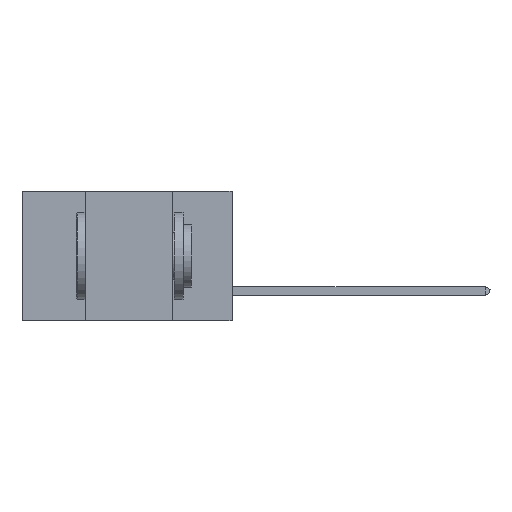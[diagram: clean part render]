
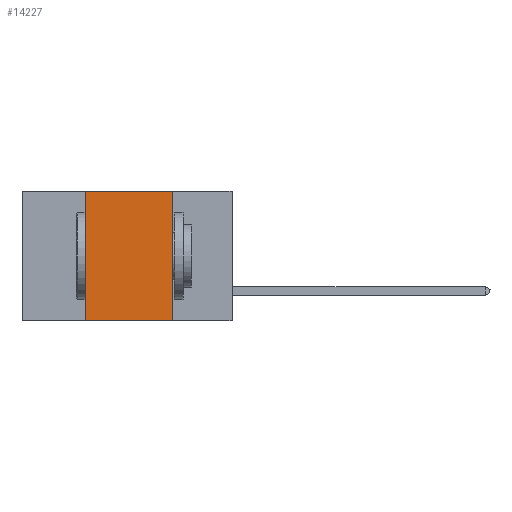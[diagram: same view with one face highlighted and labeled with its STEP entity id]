
A CAD part, left-side view. The second image highlights one B-rep face of the part: STEP entity #14227.
In plain terms, the highlighted planar face has unit normal (-1, 0, 0).
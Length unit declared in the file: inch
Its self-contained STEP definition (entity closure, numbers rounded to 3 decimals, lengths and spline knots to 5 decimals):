
#2459 = EDGE_CURVE ( 'NONE', #25816, #4849, #21942, .T. ) ;
#2851 = FACE_OUTER_BOUND ( 'NONE', #14474, .T. ) ;
#3013 = DIRECTION ( 'NONE',  ( 1., 0., 0. ) ) ;
#3848 = CARTESIAN_POINT ( 'NONE',  ( 0., 0.42, 0. ) ) ;
#4849 = VERTEX_POINT ( 'NONE', #29772 ) ;
#5055 = ORIENTED_EDGE ( 'NONE', *, *, #19666, .T. ) ;
#5591 = CARTESIAN_POINT ( 'NONE',  ( 0., 0.42, 0. ) ) ;
#6212 = CARTESIAN_POINT ( 'NONE',  ( 0., 0.6, 0. ) ) ;
#6793 = VECTOR ( 'NONE', #21826, 39.37008 ) ;
#7305 = ORIENTED_EDGE ( 'NONE', *, *, #2459, .F. ) ;
#8101 = CARTESIAN_POINT ( 'NONE',  ( 0., 0.6, 0. ) ) ;
#10508 = LINE ( 'NONE', #5591, #17459 ) ;
#13150 = PLANE ( 'NONE',  #19511 ) ;
#13334 = VERTEX_POINT ( 'NONE', #31915 ) ;
#13373 = DIRECTION ( 'NONE',  ( 0., 0., -1. ) ) ;
#13843 = DIRECTION ( 'NONE',  ( 0., -1., 0. ) ) ;
#14227 = ADVANCED_FACE ( 'NONE', ( #2851 ), #13150, .F. ) ;
#14469 = CARTESIAN_POINT ( 'NONE',  ( 0., 0.6, -0.37 ) ) ;
#14474 = EDGE_LOOP ( 'NONE', ( #30489, #7305, #22031, #5055 ) ) ;
#14906 = VECTOR ( 'NONE', #27967, 39.37008 ) ;
#15980 = CARTESIAN_POINT ( 'NONE',  ( 0., 0.17, -0.37 ) ) ;
#16137 = DIRECTION ( 'NONE',  ( 0., 0., 1. ) ) ;
#17459 = VECTOR ( 'NONE', #16137, 39.37008 ) ;
#18774 = EDGE_CURVE ( 'NONE', #4849, #26867, #21653, .T. ) ;
#19085 = EDGE_CURVE ( 'NONE', #13334, #25816, #10508, .T. ) ;
#19511 = AXIS2_PLACEMENT_3D ( 'NONE', #8101, #3013, #13373 ) ;
#19515 = LINE ( 'NONE', #14469, #25277 ) ;
#19666 = EDGE_CURVE ( 'NONE', #13334, #26867, #19515, .T. ) ;
#21653 = LINE ( 'NONE', #22286, #6793 ) ;
#21826 = DIRECTION ( 'NONE',  ( 0., 0., -1. ) ) ;
#21942 = LINE ( 'NONE', #6212, #14906 ) ;
#22031 = ORIENTED_EDGE ( 'NONE', *, *, #19085, .F. ) ;
#22286 = CARTESIAN_POINT ( 'NONE',  ( 0., 0.17, 0. ) ) ;
#25277 = VECTOR ( 'NONE', #13843, 39.37008 ) ;
#25816 = VERTEX_POINT ( 'NONE', #3848 ) ;
#26867 = VERTEX_POINT ( 'NONE', #15980 ) ;
#27967 = DIRECTION ( 'NONE',  ( 0., -1., 0. ) ) ;
#29772 = CARTESIAN_POINT ( 'NONE',  ( 0., 0.17, 0. ) ) ;
#30489 = ORIENTED_EDGE ( 'NONE', *, *, #18774, .F. ) ;
#31915 = CARTESIAN_POINT ( 'NONE',  ( 0., 0.42, -0.37 ) ) ;
